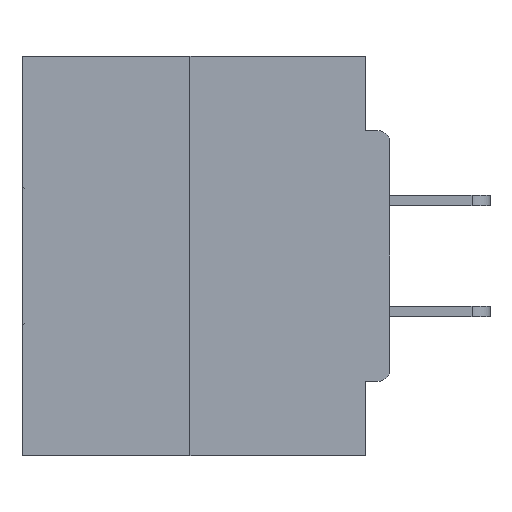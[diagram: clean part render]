
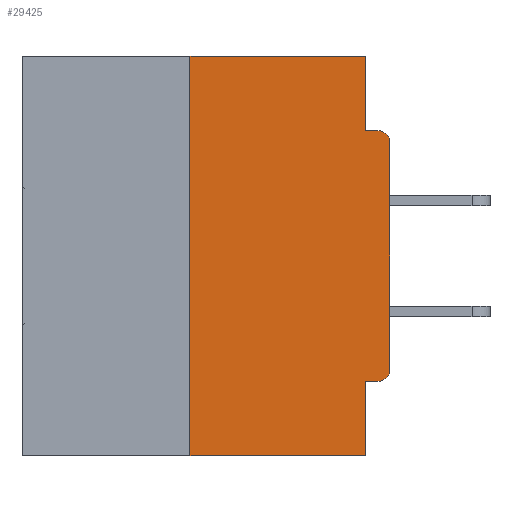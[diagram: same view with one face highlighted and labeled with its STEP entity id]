
A CAD part, left-side view. The second image highlights one B-rep face of the part: STEP entity #29425.
In plain terms, the highlighted planar face has unit normal (-1, 0, 0).
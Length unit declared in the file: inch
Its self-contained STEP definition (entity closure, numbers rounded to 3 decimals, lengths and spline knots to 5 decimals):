
#432 = ORIENTED_EDGE ( 'NONE', *, *, #32563, .T. ) ;
#1448 = ORIENTED_EDGE ( 'NONE', *, *, #32364, .F. ) ;
#2558 = CARTESIAN_POINT ( 'NONE',  ( 0., 0., -0.4065 ) ) ;
#2961 = ORIENTED_EDGE ( 'NONE', *, *, #6428, .T. ) ;
#3900 = VERTEX_POINT ( 'NONE', #12642 ) ;
#4425 = ORIENTED_EDGE ( 'NONE', *, *, #24732, .F. ) ;
#4769 = LINE ( 'NONE', #17002, #37598 ) ;
#4834 = DIRECTION ( 'NONE',  ( 0., 0., 1. ) ) ;
#5257 = VERTEX_POINT ( 'NONE', #7474 ) ;
#5362 = CARTESIAN_POINT ( 'NONE',  ( 0., 0.46, -0.5 ) ) ;
#6428 = EDGE_CURVE ( 'NONE', #37131, #3900, #4769, .T. ) ;
#6743 = CARTESIAN_POINT ( 'NONE',  ( 0., 0.25, -0.5 ) ) ;
#7474 = CARTESIAN_POINT ( 'NONE',  ( 0., 0.015, -0.0935 ) ) ;
#7768 = DIRECTION ( 'NONE',  ( 0., 0., -1. ) ) ;
#7912 = VECTOR ( 'NONE', #22269, 39.37008 ) ;
#9029 = EDGE_CURVE ( 'NONE', #16396, #5257, #18792, .T. ) ;
#9587 = VECTOR ( 'NONE', #36221, 39.37008 ) ;
#10386 = CARTESIAN_POINT ( 'NONE',  ( 0., 0.031, -0.0935 ) ) ;
#10910 = ORIENTED_EDGE ( 'NONE', *, *, #15790, .F. ) ;
#10968 = VECTOR ( 'NONE', #21919, 39.37008 ) ;
#11131 = LINE ( 'NONE', #20708, #21330 ) ;
#11764 = VERTEX_POINT ( 'NONE', #12157 ) ;
#12157 = CARTESIAN_POINT ( 'NONE',  ( 0., 0.031, -0.5 ) ) ;
#12513 = CARTESIAN_POINT ( 'NONE',  ( 0., 0.46, 0. ) ) ;
#12642 = CARTESIAN_POINT ( 'NONE',  ( 0., 0., -0.1085 ) ) ;
#14155 = ORIENTED_EDGE ( 'NONE', *, *, #16579, .F. ) ;
#14365 = AXIS2_PLACEMENT_3D ( 'NONE', #36838, #36722, #33662 ) ;
#14581 = CARTESIAN_POINT ( 'NONE',  ( 0., 0., -0.0935 ) ) ;
#14871 = VERTEX_POINT ( 'NONE', #17240 ) ;
#14980 = ORIENTED_EDGE ( 'NONE', *, *, #29241, .F. ) ;
#15038 = ORIENTED_EDGE ( 'NONE', *, *, #9029, .F. ) ;
#15237 = DIRECTION ( 'NONE',  ( 0., 0., -1. ) ) ;
#15790 = EDGE_CURVE ( 'NONE', #18340, #11764, #21671, .T. ) ;
#16155 = LINE ( 'NONE', #37605, #7912 ) ;
#16396 = VERTEX_POINT ( 'NONE', #10386 ) ;
#16417 = CARTESIAN_POINT ( 'NONE',  ( 0., 0., -0.3915 ) ) ;
#16579 = EDGE_CURVE ( 'NONE', #24907, #22160, #37025, .T. ) ;
#16776 = CIRCLE ( 'NONE', #14365, 0.015 ) ;
#17002 = CARTESIAN_POINT ( 'NONE',  ( 0., 0., 0. ) ) ;
#17240 = CARTESIAN_POINT ( 'NONE',  ( 0., 0.015, -0.4065 ) ) ;
#17613 = CARTESIAN_POINT ( 'NONE',  ( 0., 0.015, -0.1085 ) ) ;
#17881 = AXIS2_PLACEMENT_3D ( 'NONE', #17613, #26571, #7768 ) ;
#17914 = VERTEX_POINT ( 'NONE', #39464 ) ;
#18340 = VERTEX_POINT ( 'NONE', #39282 ) ;
#18622 = PLANE ( 'NONE',  #36699 ) ;
#18792 = LINE ( 'NONE', #14581, #9587 ) ;
#19390 = LINE ( 'NONE', #5362, #20832 ) ;
#19861 = EDGE_LOOP ( 'NONE', ( #4425, #14155, #39639, #10910, #14980, #34618, #2961, #432, #15038, #1448 ) ) ;
#20708 = CARTESIAN_POINT ( 'NONE',  ( 0., 0.46, 0. ) ) ;
#20832 = VECTOR ( 'NONE', #30091, 39.37008 ) ;
#21330 = VECTOR ( 'NONE', #24075, 39.37008 ) ;
#21671 = LINE ( 'NONE', #36872, #10968 ) ;
#21919 = DIRECTION ( 'NONE',  ( 0., 0., -1. ) ) ;
#22160 = VERTEX_POINT ( 'NONE', #39603 ) ;
#22269 = DIRECTION ( 'NONE',  ( 0., 0., -1. ) ) ;
#22720 = VECTOR ( 'NONE', #39144, 39.37008 ) ;
#23795 = DIRECTION ( 'NONE',  ( 0., 0., 1. ) ) ;
#24075 = DIRECTION ( 'NONE',  ( 0., -1., 0. ) ) ;
#24732 = EDGE_CURVE ( 'NONE', #22160, #17914, #11131, .T. ) ;
#24907 = VERTEX_POINT ( 'NONE', #6743 ) ;
#25633 = LINE ( 'NONE', #2558, #22720 ) ;
#25866 = CIRCLE ( 'NONE', #17881, 0.015 ) ;
#26571 = DIRECTION ( 'NONE',  ( -1., 0., 0. ) ) ;
#27147 = CARTESIAN_POINT ( 'NONE',  ( 0., 0.25, 0. ) ) ;
#27544 = FACE_OUTER_BOUND ( 'NONE', #19861, .T. ) ;
#27693 = EDGE_CURVE ( 'NONE', #14871, #37131, #16776, .T. ) ;
#29241 = EDGE_CURVE ( 'NONE', #14871, #18340, #25633, .T. ) ;
#29425 = ADVANCED_FACE ( 'NONE', ( #27544 ), #18622, .F. ) ;
#30091 = DIRECTION ( 'NONE',  ( 0., -1., 0. ) ) ;
#32364 = EDGE_CURVE ( 'NONE', #17914, #16396, #16155, .T. ) ;
#32563 = EDGE_CURVE ( 'NONE', #3900, #5257, #25866, .T. ) ;
#33202 = VECTOR ( 'NONE', #23795, 39.37008 ) ;
#33662 = DIRECTION ( 'NONE',  ( 0., 0., -1. ) ) ;
#33799 = DIRECTION ( 'NONE',  ( 1., 0., 0. ) ) ;
#34618 = ORIENTED_EDGE ( 'NONE', *, *, #27693, .T. ) ;
#35919 = EDGE_CURVE ( 'NONE', #24907, #11764, #19390, .T. ) ;
#36221 = DIRECTION ( 'NONE',  ( 0., -1., 0. ) ) ;
#36699 = AXIS2_PLACEMENT_3D ( 'NONE', #12513, #33799, #15237 ) ;
#36722 = DIRECTION ( 'NONE',  ( -1., 0., 0. ) ) ;
#36838 = CARTESIAN_POINT ( 'NONE',  ( 0., 0.015, -0.3915 ) ) ;
#36872 = CARTESIAN_POINT ( 'NONE',  ( 0., 0.031, -0.5 ) ) ;
#37025 = LINE ( 'NONE', #27147, #33202 ) ;
#37131 = VERTEX_POINT ( 'NONE', #16417 ) ;
#37598 = VECTOR ( 'NONE', #4834, 39.37008 ) ;
#37605 = CARTESIAN_POINT ( 'NONE',  ( 0., 0.031, 0. ) ) ;
#39144 = DIRECTION ( 'NONE',  ( 0., 1., 0. ) ) ;
#39282 = CARTESIAN_POINT ( 'NONE',  ( 0., 0.031, -0.4065 ) ) ;
#39464 = CARTESIAN_POINT ( 'NONE',  ( 0., 0.031, 0. ) ) ;
#39603 = CARTESIAN_POINT ( 'NONE',  ( 0., 0.25, 0. ) ) ;
#39639 = ORIENTED_EDGE ( 'NONE', *, *, #35919, .T. ) ;
